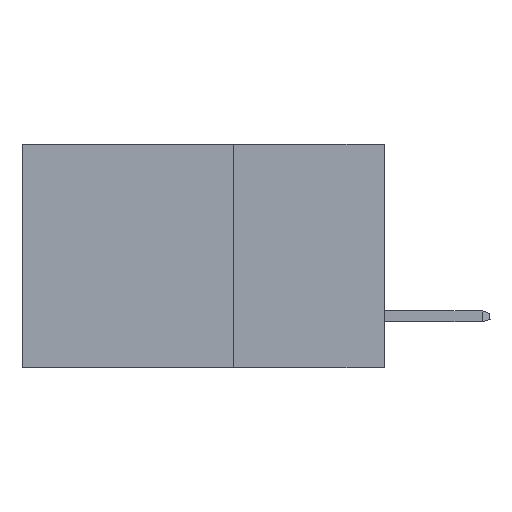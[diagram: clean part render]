
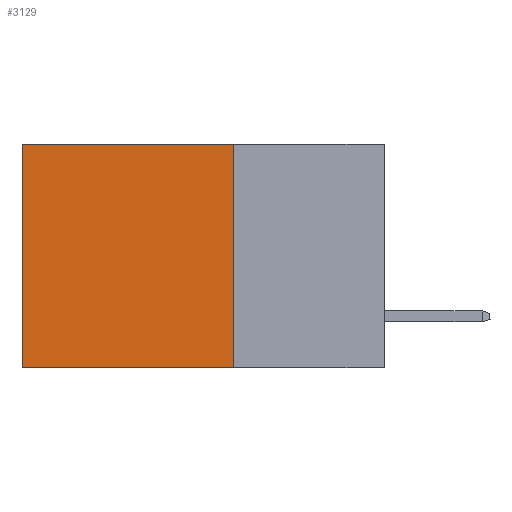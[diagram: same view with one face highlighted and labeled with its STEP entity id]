
A CAD part, left-side view. The second image highlights one B-rep face of the part: STEP entity #3129.
In plain terms, the highlighted planar face has unit normal (-1, 0, 0).
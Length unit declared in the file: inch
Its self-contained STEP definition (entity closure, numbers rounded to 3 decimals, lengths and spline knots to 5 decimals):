
#274 = CARTESIAN_POINT ( 'NONE',  ( 0.298, 0.6, 0. ) ) ;
#1372 = EDGE_CURVE ( 'NONE', #5528, #21950, #1408, .T. ) ;
#1408 = LINE ( 'NONE', #15526, #19374 ) ;
#2468 = EDGE_CURVE ( 'NONE', #19994, #22487, #25311, .T. ) ;
#3129 = ADVANCED_FACE ( 'NONE', ( #13659 ), #12757, .F. ) ;
#4277 = CARTESIAN_POINT ( 'NONE',  ( 0.298, 0.25, 0. ) ) ;
#4334 = VECTOR ( 'NONE', #16135, 39.37008 ) ;
#4658 = EDGE_LOOP ( 'NONE', ( #18417, #22300, #11703, #15025 ) ) ;
#5528 = VERTEX_POINT ( 'NONE', #8329 ) ;
#6195 = EDGE_CURVE ( 'NONE', #5528, #19994, #13326, .T. ) ;
#7124 = VECTOR ( 'NONE', #19189, 39.37008 ) ;
#7950 = DIRECTION ( 'NONE',  ( 0., 1., 0. ) ) ;
#8329 = CARTESIAN_POINT ( 'NONE',  ( 0.298, 0.25, 0. ) ) ;
#8552 = DIRECTION ( 'NONE',  ( 1., 0., 0. ) ) ;
#9704 = VECTOR ( 'NONE', #7950, 39.37008 ) ;
#11703 = ORIENTED_EDGE ( 'NONE', *, *, #6195, .F. ) ;
#12757 = PLANE ( 'NONE',  #23141 ) ;
#13326 = LINE ( 'NONE', #22617, #4334 ) ;
#13659 = FACE_OUTER_BOUND ( 'NONE', #4658, .T. ) ;
#15025 = ORIENTED_EDGE ( 'NONE', *, *, #1372, .T. ) ;
#15043 = DIRECTION ( 'NONE',  ( 0., 0., -1. ) ) ;
#15526 = CARTESIAN_POINT ( 'NONE',  ( 0.298, 0.25, 0. ) ) ;
#15625 = DIRECTION ( 'NONE',  ( 0., 1., 0. ) ) ;
#16135 = DIRECTION ( 'NONE',  ( 0., 0., -1. ) ) ;
#17189 = CARTESIAN_POINT ( 'NONE',  ( 0.298, 0.25, -0.37 ) ) ;
#18417 = ORIENTED_EDGE ( 'NONE', *, *, #22444, .T. ) ;
#18892 = CARTESIAN_POINT ( 'NONE',  ( 0.298, 0.25, -0.37 ) ) ;
#19189 = DIRECTION ( 'NONE',  ( 0., 0., -1. ) ) ;
#19374 = VECTOR ( 'NONE', #15625, 39.37008 ) ;
#19751 = LINE ( 'NONE', #274, #7124 ) ;
#19994 = VERTEX_POINT ( 'NONE', #17189 ) ;
#21136 = CARTESIAN_POINT ( 'NONE',  ( 0.298, 0.6, -0.37 ) ) ;
#21691 = CARTESIAN_POINT ( 'NONE',  ( 0.298, 0.6, 0. ) ) ;
#21950 = VERTEX_POINT ( 'NONE', #21691 ) ;
#22300 = ORIENTED_EDGE ( 'NONE', *, *, #2468, .F. ) ;
#22444 = EDGE_CURVE ( 'NONE', #21950, #22487, #19751, .T. ) ;
#22487 = VERTEX_POINT ( 'NONE', #21136 ) ;
#22617 = CARTESIAN_POINT ( 'NONE',  ( 0.298, 0.25, 0. ) ) ;
#23141 = AXIS2_PLACEMENT_3D ( 'NONE', #4277, #8552, #15043 ) ;
#25311 = LINE ( 'NONE', #18892, #9704 ) ;
